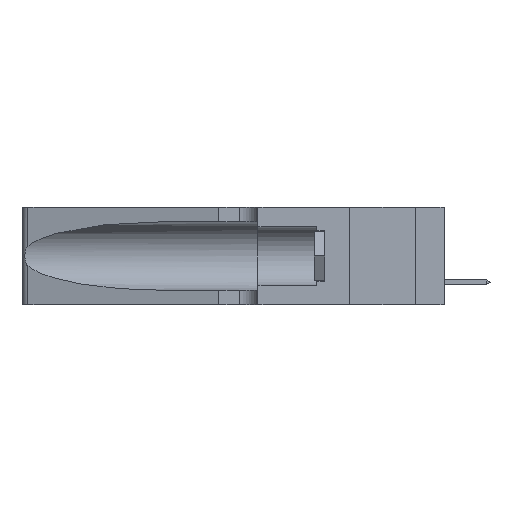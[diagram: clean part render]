
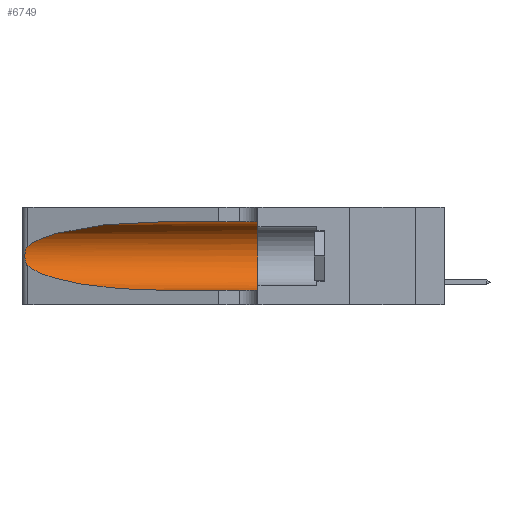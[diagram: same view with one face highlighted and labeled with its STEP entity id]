
A CAD part, left-side view. The second image highlights one B-rep face of the part: STEP entity #6749.
In plain terms, the highlighted cylindrical face has radius 3.308 mm (diameter 6.617 mm), a partial arc.
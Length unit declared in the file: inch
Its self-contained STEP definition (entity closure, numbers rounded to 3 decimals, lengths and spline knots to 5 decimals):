
#1585 = CARTESIAN_POINT ( 'NONE',  ( 0.25639, 1.23186, 0.15144 ) ) ;
#1726 = CARTESIAN_POINT ( 'NONE',  ( 0.26018, 1.23835, 0.19895 ) ) ;
#2314 =( BOUNDED_CURVE ( )  B_SPLINE_CURVE ( 3, ( #13115, #16303, #28941, #19468 ),
 .UNSPECIFIED., .F., .F. ) 
 B_SPLINE_CURVE_WITH_KNOTS ( ( 4, 4 ),
 ( 3.44316, 4.71239 ),
 .UNSPECIFIED. ) 
 CURVE ( )  GEOMETRIC_REPRESENTATION_ITEM ( )  RATIONAL_B_SPLINE_CURVE ( ( 1., 0.87, 0.87, 1. ) ) 
 REPRESENTATION_ITEM ( '' )  );
#2397 = EDGE_CURVE ( 'NONE', #37326, #3422, #31815, .T. ) ;
#2906 = ORIENTED_EDGE ( 'NONE', *, *, #2397, .F. ) ;
#3422 = VERTEX_POINT ( 'NONE', #32432 ) ;
#3749 = EDGE_CURVE ( 'NONE', #8078, #23582, #14435, .T. ) ;
#3933 = EDGE_CURVE ( 'NONE', #37326, #8078, #31594, .T. ) ;
#4946 = CARTESIAN_POINT ( 'NONE',  ( 0.1305, 1.61858, 0.31525 ) ) ;
#5471 = CARTESIAN_POINT ( 'NONE',  ( 0.25487, 1.22718, 0.22369 ) ) ;
#6675 = EDGE_CURVE ( 'NONE', #25530, #29302, #34322, .T. ) ;
#6749 = ADVANCED_FACE ( 'NONE', ( #27914 ), #12609, .F. ) ;
#7676 = CARTESIAN_POINT ( 'NONE',  ( 0.25555, 1.22994, 0.2215 ) ) ;
#7813 = CARTESIAN_POINT ( 'NONE',  ( 0.26075, 1.23896, 0.19203 ) ) ;
#7827 = CARTESIAN_POINT ( 'NONE',  ( 0.25487, 1.22718, 0.22369 ) ) ;
#8078 = VERTEX_POINT ( 'NONE', #5471 ) ;
#8767 = ORIENTED_EDGE ( 'NONE', *, *, #6675, .T. ) ;
#10416 = DIRECTION ( 'NONE',  ( 0., -1., 0. ) ) ;
#10673 = CARTESIAN_POINT ( 'NONE',  ( 0.1305, 1.61858, 0.05475 ) ) ;
#12609 = CYLINDRICAL_SURFACE ( 'NONE', #37124, 0.13025 ) ;
#13115 = CARTESIAN_POINT ( 'NONE',  ( 0.25487, 1.22718, 0.14631 ) ) ;
#13987 = CARTESIAN_POINT ( 'NONE',  ( 0.25787, 1.23484, 0.2124 ) ) ;
#14115 = CARTESIAN_POINT ( 'NONE',  ( 0.25854, 1.2359, 0.20912 ) ) ;
#14261 = CARTESIAN_POINT ( 'NONE',  ( 0.25487, 1.22718, 0.22369 ) ) ;
#14399 = CARTESIAN_POINT ( 'NONE',  ( 0.25639, 1.23184, 0.21858 ) ) ;
#14435 = B_SPLINE_CURVE_WITH_KNOTS ( 'NONE', 3,
 ( #14261, #7676, #14399, #13987, #14115, #1726, #7813, #36154, #17306, #39334, #23775, #1585, #23638, #36294 ),
 .UNSPECIFIED., .F., .F.,
 ( 4, 2, 2, 2, 2, 2, 4 ),
 ( 0., 0.00027, 0.00053, 0.00107, 0.0016, 0.00187, 0.00214 ),
 .UNSPECIFIED. ) ;
#14520 = DIRECTION ( 'NONE',  ( 0., 0., -1. ) ) ;
#14779 = DIRECTION ( 'NONE',  ( 0., 1., 0. ) ) ;
#15071 = VECTOR ( 'NONE', #36473, 39.37008 ) ;
#15196 = CARTESIAN_POINT ( 'NONE',  ( 0.1305, 0.35, 0.185 ) ) ;
#15831 = CIRCLE ( 'NONE', #32097, 0.13025 ) ;
#15842 = ORIENTED_EDGE ( 'NONE', *, *, #18733, .F. ) ;
#16303 = CARTESIAN_POINT ( 'NONE',  ( 0.2373, 1.15595, 0.08982 ) ) ;
#17306 = CARTESIAN_POINT ( 'NONE',  ( 0.26017, 1.23833, 0.17102 ) ) ;
#18566 = VECTOR ( 'NONE', #10416, 39.37008 ) ;
#18733 = EDGE_CURVE ( 'NONE', #3422, #29302, #15831, .T. ) ;
#19468 = CARTESIAN_POINT ( 'NONE',  ( 0.1305, 0.72297, 0.05475 ) ) ;
#21326 = EDGE_CURVE ( 'NONE', #23582, #25530, #2314, .T. ) ;
#22288 = CARTESIAN_POINT ( 'NONE',  ( 0.1305, 0.72297, 0.31525 ) ) ;
#23374 = CARTESIAN_POINT ( 'NONE',  ( 0.2373, 1.15595, 0.28018 ) ) ;
#23510 = CARTESIAN_POINT ( 'NONE',  ( 0.18966, 0.96281, 0.31525 ) ) ;
#23582 = VERTEX_POINT ( 'NONE', #29187 ) ;
#23638 = CARTESIAN_POINT ( 'NONE',  ( 0.25555, 1.22993, 0.14849 ) ) ;
#23775 = CARTESIAN_POINT ( 'NONE',  ( 0.25789, 1.23486, 0.15765 ) ) ;
#25530 = VERTEX_POINT ( 'NONE', #32084 ) ;
#26041 = ORIENTED_EDGE ( 'NONE', *, *, #3749, .T. ) ;
#26292 = EDGE_LOOP ( 'NONE', ( #29023, #26041, #37746, #8767, #15842, #2906 ) ) ;
#26749 = CARTESIAN_POINT ( 'NONE',  ( 0.1305, 0.72297, 0.31525 ) ) ;
#27914 = FACE_OUTER_BOUND ( 'NONE', #26292, .T. ) ;
#28941 = CARTESIAN_POINT ( 'NONE',  ( 0.18966, 0.96281, 0.05475 ) ) ;
#29023 = ORIENTED_EDGE ( 'NONE', *, *, #3933, .T. ) ;
#29187 = CARTESIAN_POINT ( 'NONE',  ( 0.25487, 1.22718, 0.14631 ) ) ;
#29302 = VERTEX_POINT ( 'NONE', #35469 ) ;
#30483 = DIRECTION ( 'NONE',  ( 0., 0., 1. ) ) ;
#31594 =( BOUNDED_CURVE ( )  B_SPLINE_CURVE ( 3, ( #22288, #23510, #23374, #7827 ),
 .UNSPECIFIED., .F., .T. ) 
 B_SPLINE_CURVE_WITH_KNOTS ( ( 4, 4 ),
 ( 1.5708, 2.84003 ),
 .UNSPECIFIED. ) 
 CURVE ( )  GEOMETRIC_REPRESENTATION_ITEM ( )  RATIONAL_B_SPLINE_CURVE ( ( 1., 0.87, 0.87, 1. ) ) 
 REPRESENTATION_ITEM ( '' )  );
#31815 = LINE ( 'NONE', #4946, #15071 ) ;
#32084 = CARTESIAN_POINT ( 'NONE',  ( 0.1305, 0.72297, 0.05475 ) ) ;
#32097 = AXIS2_PLACEMENT_3D ( 'NONE', #15196, #14779, #30483 ) ;
#32432 = CARTESIAN_POINT ( 'NONE',  ( 0.1305, 0.35, 0.31525 ) ) ;
#34322 = LINE ( 'NONE', #10673, #18566 ) ;
#35469 = CARTESIAN_POINT ( 'NONE',  ( 0.1305, 0.35, 0.05475 ) ) ;
#36154 = CARTESIAN_POINT ( 'NONE',  ( 0.26075, 1.23896, 0.178 ) ) ;
#36294 = CARTESIAN_POINT ( 'NONE',  ( 0.25487, 1.22718, 0.14631 ) ) ;
#36473 = DIRECTION ( 'NONE',  ( 0., -1., 0. ) ) ;
#37124 = AXIS2_PLACEMENT_3D ( 'NONE', #39182, #38631, #14520 ) ;
#37326 = VERTEX_POINT ( 'NONE', #26749 ) ;
#37746 = ORIENTED_EDGE ( 'NONE', *, *, #21326, .T. ) ;
#38631 = DIRECTION ( 'NONE',  ( 0., -1., 0. ) ) ;
#39182 = CARTESIAN_POINT ( 'NONE',  ( 0.1305, 1.61858, 0.185 ) ) ;
#39334 = CARTESIAN_POINT ( 'NONE',  ( 0.25856, 1.23593, 0.16098 ) ) ;
